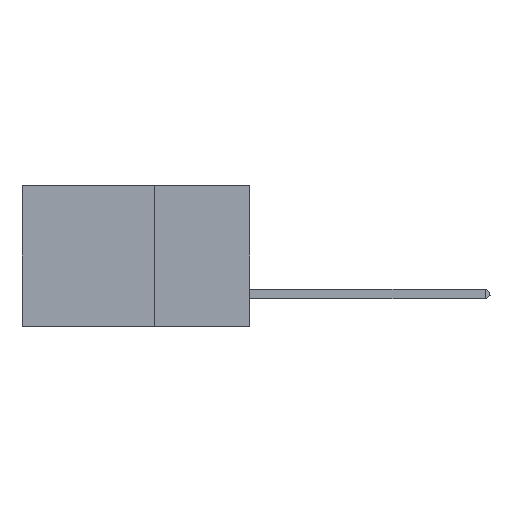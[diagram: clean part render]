
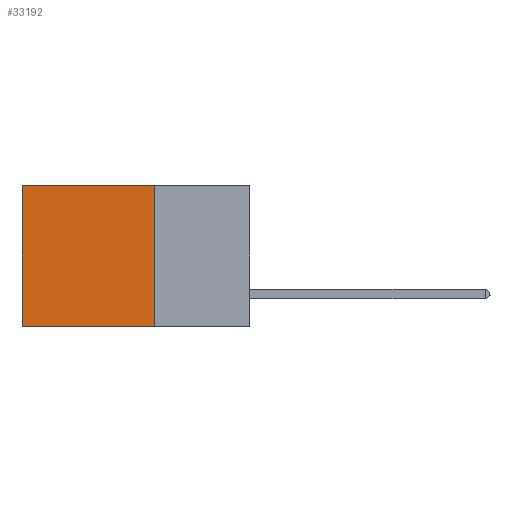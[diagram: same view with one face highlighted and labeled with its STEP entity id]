
A CAD part, left-side view. The second image highlights one B-rep face of the part: STEP entity #33192.
In plain terms, the highlighted planar face has unit normal (-1, 0, 0).
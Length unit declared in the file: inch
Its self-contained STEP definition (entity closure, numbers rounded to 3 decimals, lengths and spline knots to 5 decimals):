
#487 = ORIENTED_EDGE ( 'NONE', *, *, #25356, .T. ) ;
#962 = DIRECTION ( 'NONE',  ( 0., 1., 0. ) ) ;
#2492 = DIRECTION ( 'NONE',  ( 0., 1., 0. ) ) ;
#4633 = ORIENTED_EDGE ( 'NONE', *, *, #16196, .T. ) ;
#4870 = CARTESIAN_POINT ( 'NONE',  ( 0.2875, 0.6, -0.37 ) ) ;
#5046 = CARTESIAN_POINT ( 'NONE',  ( 0.2875, 0.25, 0. ) ) ;
#5659 = CARTESIAN_POINT ( 'NONE',  ( 0.2875, 0.25, 0. ) ) ;
#5978 = EDGE_CURVE ( 'NONE', #19103, #38804, #30692, .T. ) ;
#6504 = LINE ( 'NONE', #10940, #21599 ) ;
#6572 = DIRECTION ( 'NONE',  ( 0., 0., -1. ) ) ;
#7244 = DIRECTION ( 'NONE',  ( 0., 0., -1. ) ) ;
#9344 = EDGE_LOOP ( 'NONE', ( #4633, #21990, #21333, #487 ) ) ;
#10455 = CARTESIAN_POINT ( 'NONE',  ( 0.2875, 0.25, 0. ) ) ;
#10940 = CARTESIAN_POINT ( 'NONE',  ( 0.2875, 0.25, -0.37 ) ) ;
#11552 = VERTEX_POINT ( 'NONE', #4870 ) ;
#13476 = CARTESIAN_POINT ( 'NONE',  ( 0.2875, 0.25, -0.37 ) ) ;
#13945 = VECTOR ( 'NONE', #7244, 39.37008 ) ;
#16196 = EDGE_CURVE ( 'NONE', #23270, #11552, #30512, .T. ) ;
#19103 = VERTEX_POINT ( 'NONE', #42889 ) ;
#19583 = DIRECTION ( 'NONE',  ( 1., 0., 0. ) ) ;
#20896 = FACE_OUTER_BOUND ( 'NONE', #9344, .T. ) ;
#21333 = ORIENTED_EDGE ( 'NONE', *, *, #5978, .F. ) ;
#21599 = VECTOR ( 'NONE', #962, 39.37008 ) ;
#21990 = ORIENTED_EDGE ( 'NONE', *, *, #37153, .F. ) ;
#23270 = VERTEX_POINT ( 'NONE', #29440 ) ;
#25319 = AXIS2_PLACEMENT_3D ( 'NONE', #5659, #19583, #6572 ) ;
#25356 = EDGE_CURVE ( 'NONE', #19103, #23270, #29337, .T. ) ;
#29337 = LINE ( 'NONE', #5046, #39543 ) ;
#29440 = CARTESIAN_POINT ( 'NONE',  ( 0.2875, 0.6, 0. ) ) ;
#30512 = LINE ( 'NONE', #36449, #42804 ) ;
#30692 = LINE ( 'NONE', #10455, #13945 ) ;
#33192 = ADVANCED_FACE ( 'NONE', ( #20896 ), #33394, .F. ) ;
#33394 = PLANE ( 'NONE',  #25319 ) ;
#36449 = CARTESIAN_POINT ( 'NONE',  ( 0.2875, 0.6, 0. ) ) ;
#37153 = EDGE_CURVE ( 'NONE', #38804, #11552, #6504, .T. ) ;
#38804 = VERTEX_POINT ( 'NONE', #13476 ) ;
#39543 = VECTOR ( 'NONE', #2492, 39.37008 ) ;
#39941 = DIRECTION ( 'NONE',  ( 0., 0., -1. ) ) ;
#42804 = VECTOR ( 'NONE', #39941, 39.37008 ) ;
#42889 = CARTESIAN_POINT ( 'NONE',  ( 0.2875, 0.25, 0. ) ) ;
